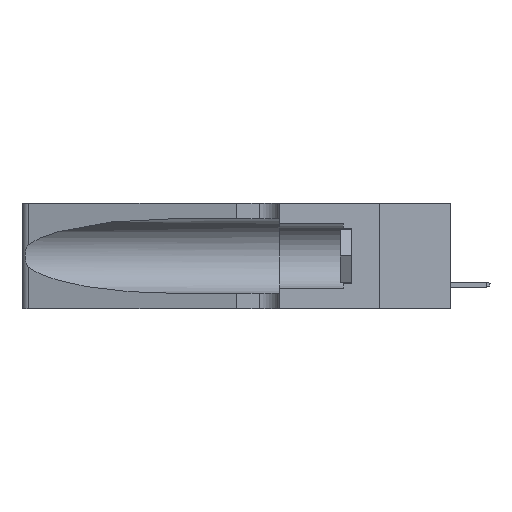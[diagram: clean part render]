
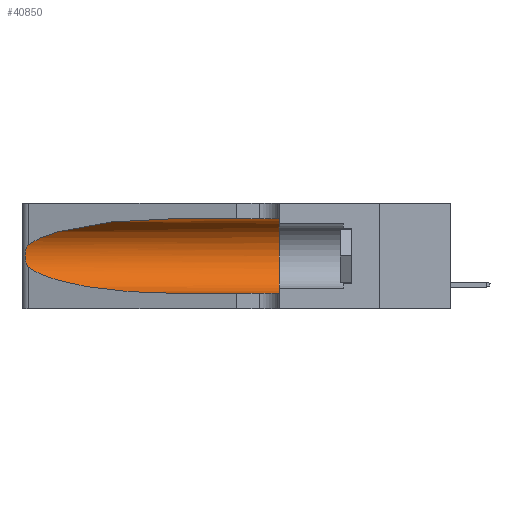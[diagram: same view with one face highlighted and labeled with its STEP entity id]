
A CAD part, left-side view. The second image highlights one B-rep face of the part: STEP entity #40850.
In plain terms, the highlighted cylindrical face has radius 3.308 mm (diameter 6.617 mm), a partial arc.
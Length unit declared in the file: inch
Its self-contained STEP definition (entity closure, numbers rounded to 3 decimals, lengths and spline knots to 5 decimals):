
#1685 = VERTEX_POINT ( 'NONE', #47655 ) ;
#2365 = AXIS2_PLACEMENT_3D ( 'NONE', #35468, #31101, #4581 ) ;
#2481 = VERTEX_POINT ( 'NONE', #32297 ) ;
#2952 = CARTESIAN_POINT ( 'NONE',  ( 0.1305, 1.61858, 0.31525 ) ) ;
#3091 = EDGE_LOOP ( 'NONE', ( #8169, #13052, #16108, #14015, #5204, #19660 ) ) ;
#3419 = CARTESIAN_POINT ( 'NONE',  ( 0.26075, 1.23896, 0.19203 ) ) ;
#3711 = DIRECTION ( 'NONE',  ( 0., -1., 0. ) ) ;
#4581 = DIRECTION ( 'NONE',  ( 0., 0., 1. ) ) ;
#5013 = VECTOR ( 'NONE', #3711, 39.37008 ) ;
#5204 = ORIENTED_EDGE ( 'NONE', *, *, #23280, .F. ) ;
#7550 = CARTESIAN_POINT ( 'NONE',  ( 0.25487, 1.22718, 0.14631 ) ) ;
#7948 = EDGE_CURVE ( 'NONE', #36214, #46954, #48188, .T. ) ;
#8169 = ORIENTED_EDGE ( 'NONE', *, *, #7948, .T. ) ;
#8815 = CYLINDRICAL_SURFACE ( 'NONE', #12395, 0.13025 ) ;
#9149 = CARTESIAN_POINT ( 'NONE',  ( 0.1305, 0.72297, 0.31525 ) ) ;
#9864 = CARTESIAN_POINT ( 'NONE',  ( 0.1305, 1.61858, 0.185 ) ) ;
#11433 = CARTESIAN_POINT ( 'NONE',  ( 0.25854, 1.2359, 0.20912 ) ) ;
#12395 = AXIS2_PLACEMENT_3D ( 'NONE', #9864, #24927, #24659 ) ;
#13052 = ORIENTED_EDGE ( 'NONE', *, *, #33570, .T. ) ;
#13053 = CARTESIAN_POINT ( 'NONE',  ( 0.1305, 0.72297, 0.05475 ) ) ;
#14015 = ORIENTED_EDGE ( 'NONE', *, *, #49512, .T. ) ;
#15302 = CARTESIAN_POINT ( 'NONE',  ( 0.26018, 1.23835, 0.19895 ) ) ;
#15905 = CARTESIAN_POINT ( 'NONE',  ( 0.2373, 1.15595, 0.08982 ) ) ;
#16108 = ORIENTED_EDGE ( 'NONE', *, *, #42575, .T. ) ;
#16153 = CARTESIAN_POINT ( 'NONE',  ( 0.18966, 0.96281, 0.31525 ) ) ;
#18968 = CARTESIAN_POINT ( 'NONE',  ( 0.25639, 1.23184, 0.21858 ) ) ;
#19052 = CARTESIAN_POINT ( 'NONE',  ( 0.25487, 1.22718, 0.14631 ) ) ;
#19216 = CARTESIAN_POINT ( 'NONE',  ( 0.26017, 1.23833, 0.17102 ) ) ;
#19660 = ORIENTED_EDGE ( 'NONE', *, *, #25547, .F. ) ;
#20832 = CARTESIAN_POINT ( 'NONE',  ( 0.1305, 1.61858, 0.05475 ) ) ;
#21112 = VECTOR ( 'NONE', #28349, 39.37008 ) ;
#22319 = CARTESIAN_POINT ( 'NONE',  ( 0.25487, 1.22718, 0.22369 ) ) ;
#23280 = EDGE_CURVE ( 'NONE', #2481, #1685, #47023, .T. ) ;
#23458 = CARTESIAN_POINT ( 'NONE',  ( 0.1305, 0.72297, 0.05475 ) ) ;
#24659 = DIRECTION ( 'NONE',  ( 0., 0., -1. ) ) ;
#24927 = DIRECTION ( 'NONE',  ( 0., -1., 0. ) ) ;
#25547 = EDGE_CURVE ( 'NONE', #36214, #2481, #31213, .T. ) ;
#26523 = CARTESIAN_POINT ( 'NONE',  ( 0.25555, 1.22994, 0.2215 ) ) ;
#28349 = DIRECTION ( 'NONE',  ( 0., -1., 0. ) ) ;
#28398 = B_SPLINE_CURVE_WITH_KNOTS ( 'NONE', 3,
 ( #38903, #26523, #18968, #42290, #11433, #15302, #3419, #30424, #19216, #31175, #42049, #38646, #46934, #7550 ),
 .UNSPECIFIED., .F., .F.,
 ( 4, 2, 2, 2, 2, 2, 4 ),
 ( 0., 0.00027, 0.00053, 0.00107, 0.0016, 0.00187, 0.00214 ),
 .UNSPECIFIED. ) ;
#30424 = CARTESIAN_POINT ( 'NONE',  ( 0.26075, 1.23896, 0.178 ) ) ;
#31006 = CARTESIAN_POINT ( 'NONE',  ( 0.18966, 0.96281, 0.05475 ) ) ;
#31101 = DIRECTION ( 'NONE',  ( 0., 1., 0. ) ) ;
#31175 = CARTESIAN_POINT ( 'NONE',  ( 0.25856, 1.23593, 0.16098 ) ) ;
#31213 = LINE ( 'NONE', #2952, #5013 ) ;
#32297 = CARTESIAN_POINT ( 'NONE',  ( 0.1305, 0.35, 0.31525 ) ) ;
#33570 = EDGE_CURVE ( 'NONE', #46954, #40929, #28398, .T. ) ;
#35468 = CARTESIAN_POINT ( 'NONE',  ( 0.1305, 0.35, 0.185 ) ) ;
#36214 = VERTEX_POINT ( 'NONE', #46017 ) ;
#38646 = CARTESIAN_POINT ( 'NONE',  ( 0.25639, 1.23186, 0.15144 ) ) ;
#38903 = CARTESIAN_POINT ( 'NONE',  ( 0.25487, 1.22718, 0.22369 ) ) ;
#40850 = ADVANCED_FACE ( 'NONE', ( #44326 ), #8815, .F. ) ;
#40929 = VERTEX_POINT ( 'NONE', #41995 ) ;
#41995 = CARTESIAN_POINT ( 'NONE',  ( 0.25487, 1.22718, 0.14631 ) ) ;
#42049 = CARTESIAN_POINT ( 'NONE',  ( 0.25789, 1.23486, 0.15765 ) ) ;
#42290 = CARTESIAN_POINT ( 'NONE',  ( 0.25787, 1.23484, 0.2124 ) ) ;
#42575 = EDGE_CURVE ( 'NONE', #40929, #50783, #47583, .T. ) ;
#43880 = CARTESIAN_POINT ( 'NONE',  ( 0.25487, 1.22718, 0.22369 ) ) ;
#44326 = FACE_OUTER_BOUND ( 'NONE', #3091, .T. ) ;
#44664 = LINE ( 'NONE', #20832, #21112 ) ;
#46017 = CARTESIAN_POINT ( 'NONE',  ( 0.1305, 0.72297, 0.31525 ) ) ;
#46934 = CARTESIAN_POINT ( 'NONE',  ( 0.25555, 1.22993, 0.14849 ) ) ;
#46954 = VERTEX_POINT ( 'NONE', #22319 ) ;
#47023 = CIRCLE ( 'NONE', #2365, 0.13025 ) ;
#47583 =( BOUNDED_CURVE ( )  B_SPLINE_CURVE ( 3, ( #19052, #15905, #31006, #23458 ),
 .UNSPECIFIED., .F., .F. ) 
 B_SPLINE_CURVE_WITH_KNOTS ( ( 4, 4 ),
 ( 3.44316, 4.71239 ),
 .UNSPECIFIED. ) 
 CURVE ( )  GEOMETRIC_REPRESENTATION_ITEM ( )  RATIONAL_B_SPLINE_CURVE ( ( 1., 0.87, 0.87, 1. ) ) 
 REPRESENTATION_ITEM ( '' )  );
#47655 = CARTESIAN_POINT ( 'NONE',  ( 0.1305, 0.35, 0.05475 ) ) ;
#48188 =( BOUNDED_CURVE ( )  B_SPLINE_CURVE ( 3, ( #9149, #16153, #48541, #43880 ),
 .UNSPECIFIED., .F., .F. ) 
 B_SPLINE_CURVE_WITH_KNOTS ( ( 4, 4 ),
 ( 1.5708, 2.84003 ),
 .UNSPECIFIED. ) 
 CURVE ( )  GEOMETRIC_REPRESENTATION_ITEM ( )  RATIONAL_B_SPLINE_CURVE ( ( 1., 0.87, 0.87, 1. ) ) 
 REPRESENTATION_ITEM ( '' )  );
#48541 = CARTESIAN_POINT ( 'NONE',  ( 0.2373, 1.15595, 0.28018 ) ) ;
#49512 = EDGE_CURVE ( 'NONE', #50783, #1685, #44664, .T. ) ;
#50783 = VERTEX_POINT ( 'NONE', #13053 ) ;
